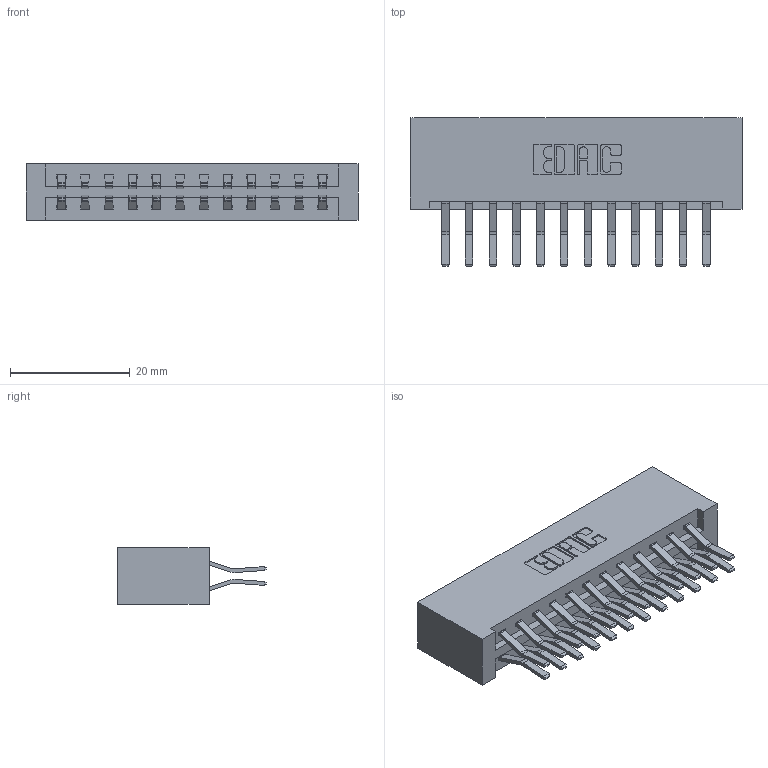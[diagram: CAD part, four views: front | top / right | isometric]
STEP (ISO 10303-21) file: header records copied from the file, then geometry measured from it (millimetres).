
FILE_DESCRIPTION (( 'STEP AP203' ), '1' );
FILE_NAME ('337-024-560-201.STEP', '2019-10-08T15:48:34', ( '' ), ( '' ), 'SwSTEP 2.0', 'SolidWorks 2016', '' );
FILE_SCHEMA (( 'CONFIG_CONTROL_DESIGN' ));
Length unit declared in the file: inch
Products named in the file (3): 337 Part_No Mounting Lugs; 345-292-001_560 Tail; 337-024-560-201
Assembly tree (25 placements, depth 2):
  337-024-560-201
    337 Part_No Mounting Lugs
    345-292-001_560 Tail  x24
Bounding box: 55.42 x 24.78 x 9.4 mm (x, y, z)
Volume: 6359.6 mm3; surface area: 7409.5 mm2
Topology: 25 solids, 25 shells, 1450 faces, 4295 edges, 2830 vertices
Faces by surface type: plane 978, cylinder 472
Entity records: 12995 total; most frequent: CARTESIAN_POINT 2214, ORIENTED_EDGE 2150, DIRECTION 1935, EDGE_CURVE 1075, VECTOR 951, LINE 951, VERTEX_POINT 714, AXIS2_PLACEMENT_3D 492
